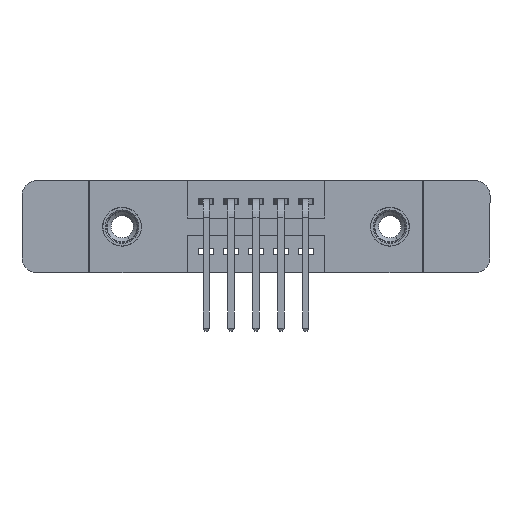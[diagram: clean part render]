
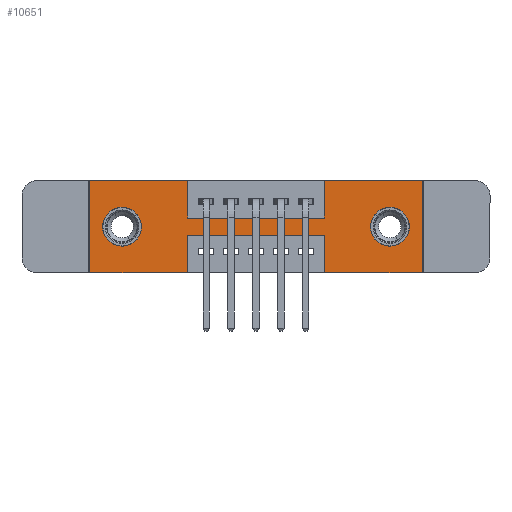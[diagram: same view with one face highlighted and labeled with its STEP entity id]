
A CAD part, front view. The second image highlights one B-rep face of the part: STEP entity #10651.
In plain terms, the highlighted planar face has unit normal (0, -1, 0).
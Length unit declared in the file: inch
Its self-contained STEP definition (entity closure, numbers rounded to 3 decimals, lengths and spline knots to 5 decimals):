
#60 = CARTESIAN_POINT ( 'NONE',  ( 0.3925, 0., -0.37 ) ) ;
#152 = CIRCLE ( 'NONE', #5830, 0.078 ) ;
#162 = CIRCLE ( 'NONE', #3188, 0.078 ) ;
#165 = DIRECTION ( 'NONE',  ( 0., 1., 0. ) ) ;
#289 = CARTESIAN_POINT ( 'NONE',  ( 0., 0., 0. ) ) ;
#323 = ORIENTED_EDGE ( 'NONE', *, *, #12143, .T. ) ;
#407 = EDGE_CURVE ( 'NONE', #9489, #12733, #12478, .T. ) ;
#466 = CARTESIAN_POINT ( 'NONE',  ( 0.9425, 0., 0. ) ) ;
#476 = CARTESIAN_POINT ( 'NONE',  ( 0.9425, 0., -0.22 ) ) ;
#622 = DIRECTION ( 'NONE',  ( 0., 0., 1. ) ) ;
#769 = VERTEX_POINT ( 'NONE', #466 ) ;
#841 = CARTESIAN_POINT ( 'NONE',  ( 1.205, 0., -0.107 ) ) ;
#1067 = AXIS2_PLACEMENT_3D ( 'NONE', #3825, #11437, #4912 ) ;
#1098 = VECTOR ( 'NONE', #12142, 39.37008 ) ;
#1316 = CARTESIAN_POINT ( 'NONE',  ( 1.335, 0., 0. ) ) ;
#1610 = DIRECTION ( 'NONE',  ( 0., -1., 0. ) ) ;
#1676 = VERTEX_POINT ( 'NONE', #60 ) ;
#1919 = VERTEX_POINT ( 'NONE', #13466 ) ;
#1989 = CARTESIAN_POINT ( 'NONE',  ( 0.3925, 0., 0. ) ) ;
#2022 = ORIENTED_EDGE ( 'NONE', *, *, #11419, .F. ) ;
#2430 = VECTOR ( 'NONE', #4385, 39.37008 ) ;
#2562 = ORIENTED_EDGE ( 'NONE', *, *, #3816, .F. ) ;
#2591 = VECTOR ( 'NONE', #4323, 39.37008 ) ;
#2659 = LINE ( 'NONE', #289, #13834 ) ;
#2674 = LINE ( 'NONE', #1989, #11332 ) ;
#2768 = EDGE_CURVE ( 'NONE', #8354, #769, #8049, .T. ) ;
#2967 = FACE_OUTER_BOUND ( 'NONE', #10142, .T. ) ;
#3188 = AXIS2_PLACEMENT_3D ( 'NONE', #13556, #7097, #622 ) ;
#3201 = VERTEX_POINT ( 'NONE', #9518 ) ;
#3235 = CARTESIAN_POINT ( 'NONE',  ( 0.9425, 0., 0. ) ) ;
#3282 = ORIENTED_EDGE ( 'NONE', *, *, #3757, .F. ) ;
#3461 = CARTESIAN_POINT ( 'NONE',  ( 0.13, 0., -0.107 ) ) ;
#3546 = VECTOR ( 'NONE', #5941, 39.37008 ) ;
#3605 = DIRECTION ( 'NONE',  ( 0., 0., -1. ) ) ;
#3757 = EDGE_CURVE ( 'NONE', #12733, #10614, #7328, .T. ) ;
#3816 = EDGE_CURVE ( 'NONE', #1676, #3201, #12384, .T. ) ;
#3825 = CARTESIAN_POINT ( 'NONE',  ( 1.205, 0., -0.185 ) ) ;
#3826 = VECTOR ( 'NONE', #11792, 39.37008 ) ;
#4080 = VECTOR ( 'NONE', #8930, 39.37008 ) ;
#4153 = DIRECTION ( 'NONE',  ( 0., 0., 1. ) ) ;
#4323 = DIRECTION ( 'NONE',  ( 0., 0., 1. ) ) ;
#4385 = DIRECTION ( 'NONE',  ( 1., 0., 0. ) ) ;
#4548 = VERTEX_POINT ( 'NONE', #13456 ) ;
#4559 = EDGE_CURVE ( 'NONE', #10614, #12499, #6459, .T. ) ;
#4573 = CARTESIAN_POINT ( 'NONE',  ( 0., 0., -0.37 ) ) ;
#4640 = EDGE_CURVE ( 'NONE', #10850, #4548, #5422, .T. ) ;
#4645 = VERTEX_POINT ( 'NONE', #10420 ) ;
#4779 = ORIENTED_EDGE ( 'NONE', *, *, #4559, .F. ) ;
#4849 = ORIENTED_EDGE ( 'NONE', *, *, #12252, .F. ) ;
#4912 = DIRECTION ( 'NONE',  ( 0., 0., -1. ) ) ;
#5099 = VECTOR ( 'NONE', #4153, 39.37008 ) ;
#5133 = VECTOR ( 'NONE', #5999, 39.37008 ) ;
#5156 = DIRECTION ( 'NONE',  ( 1., 0., 0. ) ) ;
#5337 = CARTESIAN_POINT ( 'NONE',  ( 0., 0., -0.37 ) ) ;
#5422 = CIRCLE ( 'NONE', #10455, 0.078 ) ;
#5830 = AXIS2_PLACEMENT_3D ( 'NONE', #6671, #165, #7769 ) ;
#5855 = FACE_BOUND ( 'NONE', #13142, .T. ) ;
#5921 = EDGE_CURVE ( 'NONE', #12499, #1676, #10520, .T. ) ;
#5924 = ORIENTED_EDGE ( 'NONE', *, *, #4640, .T. ) ;
#5941 = DIRECTION ( 'NONE',  ( -1., 0., 0. ) ) ;
#5999 = DIRECTION ( 'NONE',  ( 1., 0., 0. ) ) ;
#6029 = AXIS2_PLACEMENT_3D ( 'NONE', #8110, #1610, #9213 ) ;
#6088 = CARTESIAN_POINT ( 'NONE',  ( 1.205, 0., -0.185 ) ) ;
#6158 = CIRCLE ( 'NONE', #1067, 0.078 ) ;
#6459 = LINE ( 'NONE', #10274, #3546 ) ;
#6671 = CARTESIAN_POINT ( 'NONE',  ( 0.13, 0., -0.185 ) ) ;
#7026 = EDGE_CURVE ( 'NONE', #13068, #9492, #162, .T. ) ;
#7097 = DIRECTION ( 'NONE',  ( 0., 1., 0. ) ) ;
#7183 = DIRECTION ( 'NONE',  ( 0., 0., -1. ) ) ;
#7228 = CARTESIAN_POINT ( 'NONE',  ( 0.3925, 0., 0. ) ) ;
#7328 = LINE ( 'NONE', #11757, #5099 ) ;
#7371 = ORIENTED_EDGE ( 'NONE', *, *, #2768, .F. ) ;
#7475 = EDGE_CURVE ( 'NONE', #9492, #13068, #152, .T. ) ;
#7632 = ORIENTED_EDGE ( 'NONE', *, *, #8446, .F. ) ;
#7640 = ORIENTED_EDGE ( 'NONE', *, *, #8726, .F. ) ;
#7643 = VECTOR ( 'NONE', #3605, 39.37008 ) ;
#7704 = LINE ( 'NONE', #12730, #13417 ) ;
#7750 = CARTESIAN_POINT ( 'NONE',  ( 0.3925, 0., -0.22 ) ) ;
#7769 = DIRECTION ( 'NONE',  ( 0., 0., 1. ) ) ;
#7786 = VERTEX_POINT ( 'NONE', #7228 ) ;
#7956 = CARTESIAN_POINT ( 'NONE',  ( 0.3925, 0., -0.37 ) ) ;
#8049 = LINE ( 'NONE', #3235, #2591 ) ;
#8110 = CARTESIAN_POINT ( 'NONE',  ( 0., 0., -0.37 ) ) ;
#8165 = ORIENTED_EDGE ( 'NONE', *, *, #5921, .F. ) ;
#8354 = VERTEX_POINT ( 'NONE', #8840 ) ;
#8404 = LINE ( 'NONE', #12471, #5133 ) ;
#8446 = EDGE_CURVE ( 'NONE', #3201, #1919, #2659, .T. ) ;
#8513 = DIRECTION ( 'NONE',  ( 0., 0., -1. ) ) ;
#8715 = ORIENTED_EDGE ( 'NONE', *, *, #407, .F. ) ;
#8726 = EDGE_CURVE ( 'NONE', #7786, #4645, #2674, .T. ) ;
#8816 = CARTESIAN_POINT ( 'NONE',  ( 0.13, 0., -0.263 ) ) ;
#8840 = CARTESIAN_POINT ( 'NONE',  ( 0.9425, 0., -0.15 ) ) ;
#8930 = DIRECTION ( 'NONE',  ( -1., 0., 0. ) ) ;
#9213 = DIRECTION ( 'NONE',  ( 0., 0., -1. ) ) ;
#9489 = VERTEX_POINT ( 'NONE', #9953 ) ;
#9492 = VERTEX_POINT ( 'NONE', #3461 ) ;
#9518 = CARTESIAN_POINT ( 'NONE',  ( 0., 0., -0.37 ) ) ;
#9813 = EDGE_LOOP ( 'NONE', ( #5924, #323 ) ) ;
#9822 = CARTESIAN_POINT ( 'NONE',  ( 0., 0., 0. ) ) ;
#9953 = CARTESIAN_POINT ( 'NONE',  ( 1.335, 0., -0.37 ) ) ;
#10071 = DIRECTION ( 'NONE',  ( 0., 0., 1. ) ) ;
#10142 = EDGE_LOOP ( 'NONE', ( #8165, #4779, #3282, #8715, #12289, #4849, #7371, #13992, #7640, #2022, #7632, #2562 ) ) ;
#10274 = CARTESIAN_POINT ( 'NONE',  ( 0.3925, 0., -0.22 ) ) ;
#10420 = CARTESIAN_POINT ( 'NONE',  ( 0.3925, 0., -0.15 ) ) ;
#10455 = AXIS2_PLACEMENT_3D ( 'NONE', #6088, #13639, #7183 ) ;
#10520 = LINE ( 'NONE', #7956, #7643 ) ;
#10614 = VERTEX_POINT ( 'NONE', #476 ) ;
#10651 = ADVANCED_FACE ( 'NONE', ( #12614, #5855, #2967 ), #13463, .T. ) ;
#10850 = VERTEX_POINT ( 'NONE', #841 ) ;
#11101 = LINE ( 'NONE', #9822, #2430 ) ;
#11202 = VERTEX_POINT ( 'NONE', #11511 ) ;
#11332 = VECTOR ( 'NONE', #8513, 39.37008 ) ;
#11419 = EDGE_CURVE ( 'NONE', #1919, #7786, #11101, .T. ) ;
#11437 = DIRECTION ( 'NONE',  ( 0., 1., 0. ) ) ;
#11511 = CARTESIAN_POINT ( 'NONE',  ( 1.335, 0., 0. ) ) ;
#11543 = EDGE_CURVE ( 'NONE', #11202, #9489, #12258, .T. ) ;
#11679 = EDGE_CURVE ( 'NONE', #4645, #8354, #8404, .T. ) ;
#11757 = CARTESIAN_POINT ( 'NONE',  ( 0.9425, 0., -0.37 ) ) ;
#11792 = DIRECTION ( 'NONE',  ( -1., 0., 0. ) ) ;
#12142 = DIRECTION ( 'NONE',  ( 0., 0., -1. ) ) ;
#12143 = EDGE_CURVE ( 'NONE', #4548, #10850, #6158, .T. ) ;
#12252 = EDGE_CURVE ( 'NONE', #769, #11202, #7704, .T. ) ;
#12258 = LINE ( 'NONE', #1316, #1098 ) ;
#12289 = ORIENTED_EDGE ( 'NONE', *, *, #11543, .F. ) ;
#12368 = ORIENTED_EDGE ( 'NONE', *, *, #7475, .T. ) ;
#12384 = LINE ( 'NONE', #4573, #4080 ) ;
#12471 = CARTESIAN_POINT ( 'NONE',  ( 0.3925, 0., -0.15 ) ) ;
#12478 = LINE ( 'NONE', #5337, #3826 ) ;
#12484 = CARTESIAN_POINT ( 'NONE',  ( 0.9425, 0., -0.37 ) ) ;
#12499 = VERTEX_POINT ( 'NONE', #7750 ) ;
#12561 = ORIENTED_EDGE ( 'NONE', *, *, #7026, .T. ) ;
#12614 = FACE_BOUND ( 'NONE', #9813, .T. ) ;
#12730 = CARTESIAN_POINT ( 'NONE',  ( 0., 0., 0. ) ) ;
#12733 = VERTEX_POINT ( 'NONE', #12484 ) ;
#13068 = VERTEX_POINT ( 'NONE', #8816 ) ;
#13142 = EDGE_LOOP ( 'NONE', ( #12368, #12561 ) ) ;
#13417 = VECTOR ( 'NONE', #5156, 39.37008 ) ;
#13456 = CARTESIAN_POINT ( 'NONE',  ( 1.205, 0., -0.263 ) ) ;
#13463 = PLANE ( 'NONE',  #6029 ) ;
#13466 = CARTESIAN_POINT ( 'NONE',  ( 0., 0., 0. ) ) ;
#13556 = CARTESIAN_POINT ( 'NONE',  ( 0.13, 0., -0.185 ) ) ;
#13639 = DIRECTION ( 'NONE',  ( 0., 1., 0. ) ) ;
#13834 = VECTOR ( 'NONE', #10071, 39.37008 ) ;
#13992 = ORIENTED_EDGE ( 'NONE', *, *, #11679, .F. ) ;
